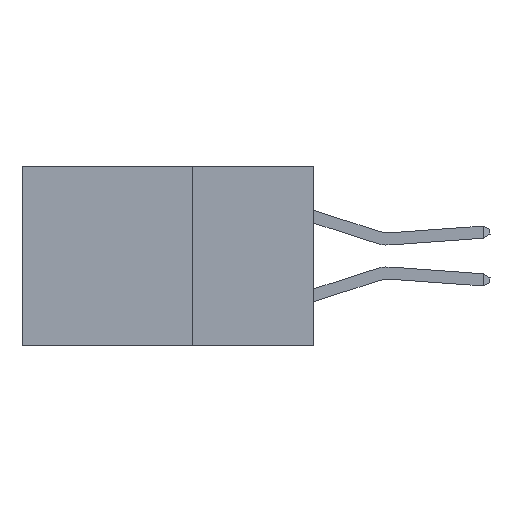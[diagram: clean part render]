
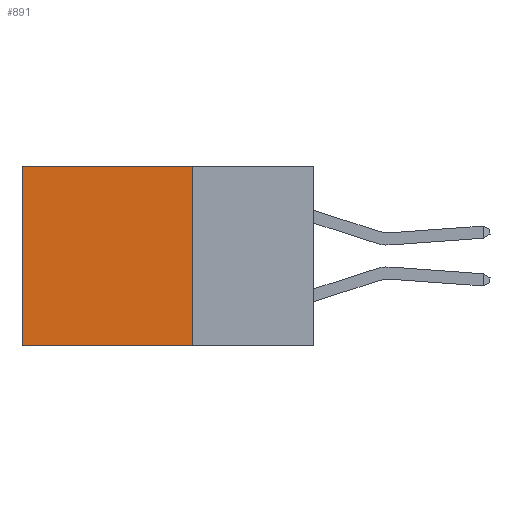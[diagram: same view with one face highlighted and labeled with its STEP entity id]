
A CAD part, left-side view. The second image highlights one B-rep face of the part: STEP entity #891.
In plain terms, the highlighted planar face has unit normal (-1, 0, 0).
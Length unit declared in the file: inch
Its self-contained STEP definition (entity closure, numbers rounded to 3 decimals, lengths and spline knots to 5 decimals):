
#417 = LINE ( 'NONE', #6356, #7219 ) ;
#891 = ADVANCED_FACE ( 'NONE', ( #11144 ), #26411, .F. ) ;
#1299 = EDGE_CURVE ( 'NONE', #28087, #7537, #26224, .T. ) ;
#1861 = ORIENTED_EDGE ( 'NONE', *, *, #13248, .T. ) ;
#2177 = CARTESIAN_POINT ( 'NONE',  ( 0.2875, 0.25, 0. ) ) ;
#3350 = VECTOR ( 'NONE', #4353, 39.37008 ) ;
#4353 = DIRECTION ( 'NONE',  ( 0., 0., -1. ) ) ;
#4592 = CARTESIAN_POINT ( 'NONE',  ( 0.2875, 0.25, 0. ) ) ;
#5080 = DIRECTION ( 'NONE',  ( 0., 1., 0. ) ) ;
#5914 = DIRECTION ( 'NONE',  ( 0., 0., -1. ) ) ;
#6356 = CARTESIAN_POINT ( 'NONE',  ( 0.2875, 0.25, -0.37 ) ) ;
#7219 = VECTOR ( 'NONE', #26502, 39.37008 ) ;
#7537 = VERTEX_POINT ( 'NONE', #22443 ) ;
#8653 = AXIS2_PLACEMENT_3D ( 'NONE', #25489, #25054, #24953 ) ;
#9098 = EDGE_CURVE ( 'NONE', #7537, #26384, #417, .T. ) ;
#11144 = FACE_OUTER_BOUND ( 'NONE', #26191, .T. ) ;
#13248 = EDGE_CURVE ( 'NONE', #28087, #23674, #36463, .T. ) ;
#13946 = VECTOR ( 'NONE', #5080, 39.37008 ) ;
#17460 = ORIENTED_EDGE ( 'NONE', *, *, #29924, .T. ) ;
#17465 = CARTESIAN_POINT ( 'NONE',  ( 0.2875, 0.6, 0. ) ) ;
#17694 = LINE ( 'NONE', #17465, #24316 ) ;
#18530 = ORIENTED_EDGE ( 'NONE', *, *, #9098, .F. ) ;
#22443 = CARTESIAN_POINT ( 'NONE',  ( 0.2875, 0.25, -0.37 ) ) ;
#23674 = VERTEX_POINT ( 'NONE', #26848 ) ;
#24316 = VECTOR ( 'NONE', #5914, 39.37008 ) ;
#24953 = DIRECTION ( 'NONE',  ( 0., 0., -1. ) ) ;
#25054 = DIRECTION ( 'NONE',  ( 1., 0., 0. ) ) ;
#25489 = CARTESIAN_POINT ( 'NONE',  ( 0.2875, 0.25, 0. ) ) ;
#26191 = EDGE_LOOP ( 'NONE', ( #17460, #18530, #35183, #1861 ) ) ;
#26224 = LINE ( 'NONE', #4592, #3350 ) ;
#26384 = VERTEX_POINT ( 'NONE', #34005 ) ;
#26411 = PLANE ( 'NONE',  #8653 ) ;
#26502 = DIRECTION ( 'NONE',  ( 0., 1., 0. ) ) ;
#26848 = CARTESIAN_POINT ( 'NONE',  ( 0.2875, 0.6, 0. ) ) ;
#28087 = VERTEX_POINT ( 'NONE', #29952 ) ;
#29924 = EDGE_CURVE ( 'NONE', #23674, #26384, #17694, .T. ) ;
#29952 = CARTESIAN_POINT ( 'NONE',  ( 0.2875, 0.25, 0. ) ) ;
#34005 = CARTESIAN_POINT ( 'NONE',  ( 0.2875, 0.6, -0.37 ) ) ;
#35183 = ORIENTED_EDGE ( 'NONE', *, *, #1299, .F. ) ;
#36463 = LINE ( 'NONE', #2177, #13946 ) ;
